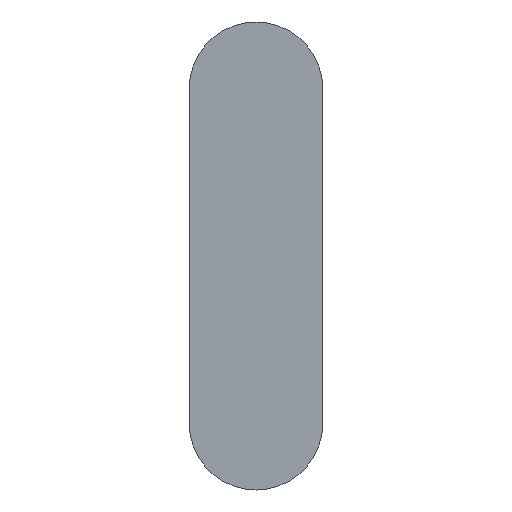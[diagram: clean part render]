
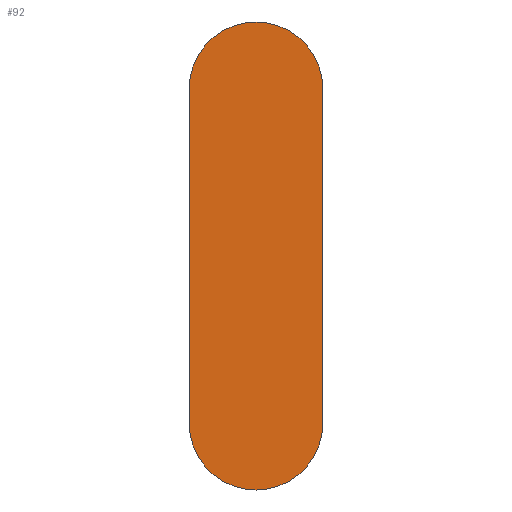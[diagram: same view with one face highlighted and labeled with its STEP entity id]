
A CAD part, front view. The second image highlights one B-rep face of the part: STEP entity #92.
In plain terms, the highlighted planar face has unit normal (0, -1, 0).
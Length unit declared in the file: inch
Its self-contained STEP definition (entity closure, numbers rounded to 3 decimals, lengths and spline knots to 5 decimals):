
#11 = CARTESIAN_POINT ( 'NONE',  ( 0., 0., -1.9685 ) ) ;
#12 = ORIENTED_EDGE ( 'NONE', *, *, #407, .F. ) ;
#14 = DIRECTION ( 'NONE',  ( 0., 1., 0. ) ) ;
#15 = DIRECTION ( 'NONE',  ( 0., 0., -1. ) ) ;
#18 = LINE ( 'NONE', #403, #159 ) ;
#30 = CARTESIAN_POINT ( 'NONE',  ( -0.3937, 0., 0. ) ) ;
#46 = DIRECTION ( 'NONE',  ( 0., 0., 1. ) ) ;
#56 = PLANE ( 'NONE',  #349 ) ;
#65 = CARTESIAN_POINT ( 'NONE',  ( 0.3937, 0., 0. ) ) ;
#76 = DIRECTION ( 'NONE',  ( 0., 1., 0. ) ) ;
#80 = VERTEX_POINT ( 'NONE', #30 ) ;
#86 = CARTESIAN_POINT ( 'NONE',  ( 0., 0., 0. ) ) ;
#92 = ADVANCED_FACE ( 'NONE', ( #278 ), #56, .F. ) ;
#129 = CIRCLE ( 'NONE', #258, 0.3937 ) ;
#132 = CARTESIAN_POINT ( 'NONE',  ( -0.3937, 0., 0. ) ) ;
#139 = DIRECTION ( 'NONE',  ( 0., 0., 1. ) ) ;
#140 = CARTESIAN_POINT ( 'NONE',  ( -0.3937, 0., -1.9685 ) ) ;
#150 = CIRCLE ( 'NONE', #149, 0.3937 ) ;
#149 = AXIS2_PLACEMENT_3D ( 'NONE', #246, #76, #286 ) ;
#156 = VERTEX_POINT ( 'NONE', #140 ) ;
#159 = VECTOR ( 'NONE', #15, 39.37008 ) ;
#160 = CARTESIAN_POINT ( 'NONE',  ( 0., 0., -2.3622 ) ) ;
#166 = ORIENTED_EDGE ( 'NONE', *, *, #397, .F. ) ;
#172 = EDGE_LOOP ( 'NONE', ( #303, #354, #363, #12, #166 ) ) ;
#188 = CARTESIAN_POINT ( 'NONE',  ( 0., 0., 0. ) ) ;
#201 = VECTOR ( 'NONE', #330, 39.37008 ) ;
#217 = DIRECTION ( 'NONE',  ( 0., 1., 0. ) ) ;
#219 = DIRECTION ( 'NONE',  ( 0., 0., 1. ) ) ;
#244 = VERTEX_POINT ( 'NONE', #384 ) ;
#246 = CARTESIAN_POINT ( 'NONE',  ( 0., 0., -1.9685 ) ) ;
#258 = AXIS2_PLACEMENT_3D ( 'NONE', #188, #14, #219 ) ;
#269 = CIRCLE ( 'NONE', #298, 0.3937 ) ;
#278 = FACE_OUTER_BOUND ( 'NONE', #172, .T. ) ;
#281 = LINE ( 'NONE', #132, #201 ) ;
#286 = DIRECTION ( 'NONE',  ( 0., 0., 1. ) ) ;
#298 = AXIS2_PLACEMENT_3D ( 'NONE', #11, #217, #46 ) ;
#303 = ORIENTED_EDGE ( 'NONE', *, *, #391, .F. ) ;
#330 = DIRECTION ( 'NONE',  ( 0., 0., 1. ) ) ;
#341 = DIRECTION ( 'NONE',  ( 0., 1., 0. ) ) ;
#348 = VERTEX_POINT ( 'NONE', #65 ) ;
#349 = AXIS2_PLACEMENT_3D ( 'NONE', #86, #341, #139 ) ;
#354 = ORIENTED_EDGE ( 'NONE', *, *, #412, .F. ) ;
#363 = ORIENTED_EDGE ( 'NONE', *, *, #383, .F. ) ;
#383 = EDGE_CURVE ( 'NONE', #418, #156, #269, .T. ) ;
#384 = CARTESIAN_POINT ( 'NONE',  ( 0.3937, 0., -1.9685 ) ) ;
#391 = EDGE_CURVE ( 'NONE', #80, #348, #129, .T. ) ;
#397 = EDGE_CURVE ( 'NONE', #348, #244, #18, .T. ) ;
#403 = CARTESIAN_POINT ( 'NONE',  ( 0.3937, 0., 0. ) ) ;
#407 = EDGE_CURVE ( 'NONE', #244, #418, #150, .T. ) ;
#412 = EDGE_CURVE ( 'NONE', #156, #80, #281, .T. ) ;
#418 = VERTEX_POINT ( 'NONE', #160 ) ;
